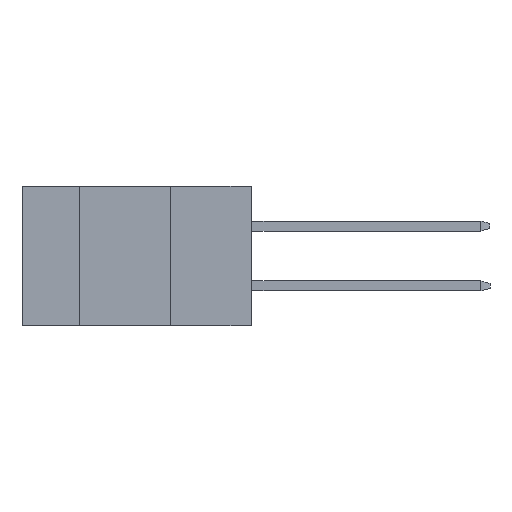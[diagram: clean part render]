
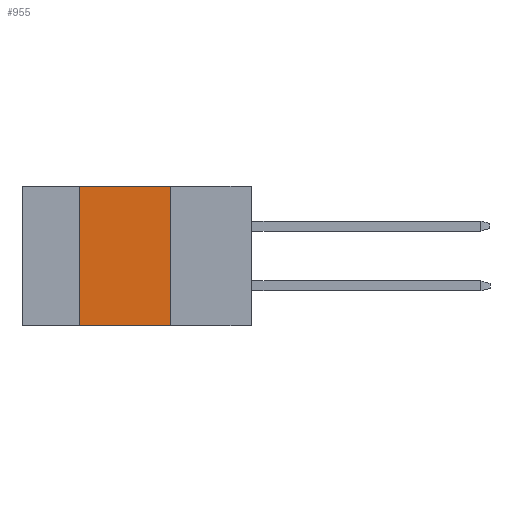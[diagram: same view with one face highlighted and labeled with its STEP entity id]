
A CAD part, left-side view. The second image highlights one B-rep face of the part: STEP entity #955.
In plain terms, the highlighted planar face has unit normal (-1, 0, 0).
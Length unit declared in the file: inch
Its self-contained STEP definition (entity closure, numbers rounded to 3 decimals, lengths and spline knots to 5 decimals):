
#553 = CARTESIAN_POINT ( 'NONE',  ( 0., 0.72, 0. ) ) ;
#832 = CARTESIAN_POINT ( 'NONE',  ( 0., 0.54, 0. ) ) ;
#886 = ORIENTED_EDGE ( 'NONE', *, *, #18858, .F. ) ;
#948 = VECTOR ( 'NONE', #7452, 39.37008 ) ;
#955 = ADVANCED_FACE ( 'NONE', ( #5339 ), #12998, .F. ) ;
#1209 = VECTOR ( 'NONE', #9947, 39.37008 ) ;
#1805 = CARTESIAN_POINT ( 'NONE',  ( 0., 0.72, -0.437 ) ) ;
#2379 = DIRECTION ( 'NONE',  ( 0., 0., -1. ) ) ;
#3817 = DIRECTION ( 'NONE',  ( 1., 0., 0. ) ) ;
#5339 = FACE_OUTER_BOUND ( 'NONE', #17587, .T. ) ;
#6115 = LINE ( 'NONE', #17029, #948 ) ;
#6169 = CARTESIAN_POINT ( 'NONE',  ( 0., 0.254, -0.437 ) ) ;
#6450 = CARTESIAN_POINT ( 'NONE',  ( 0., 0.254, 0. ) ) ;
#6986 = ORIENTED_EDGE ( 'NONE', *, *, #19279, .F. ) ;
#7402 = CARTESIAN_POINT ( 'NONE',  ( 0., 0.54, -0.437 ) ) ;
#7452 = DIRECTION ( 'NONE',  ( 0., 0., 1. ) ) ;
#7473 = DIRECTION ( 'NONE',  ( 0., 0., -1. ) ) ;
#8371 = AXIS2_PLACEMENT_3D ( 'NONE', #13296, #3817, #2379 ) ;
#8615 = EDGE_CURVE ( 'NONE', #10227, #19794, #9450, .T. ) ;
#8913 = CARTESIAN_POINT ( 'NONE',  ( 0., 0.254, -0.437 ) ) ;
#9450 = LINE ( 'NONE', #1805, #16130 ) ;
#9947 = DIRECTION ( 'NONE',  ( 0., -1., 0. ) ) ;
#10227 = VERTEX_POINT ( 'NONE', #7402 ) ;
#10707 = ORIENTED_EDGE ( 'NONE', *, *, #17778, .F. ) ;
#11055 = VERTEX_POINT ( 'NONE', #6450 ) ;
#12347 = VECTOR ( 'NONE', #7473, 39.37008 ) ;
#12717 = VERTEX_POINT ( 'NONE', #832 ) ;
#12998 = PLANE ( 'NONE',  #8371 ) ;
#13296 = CARTESIAN_POINT ( 'NONE',  ( 0., 0.72, 0. ) ) ;
#14045 = DIRECTION ( 'NONE',  ( 0., -1., 0. ) ) ;
#14528 = LINE ( 'NONE', #553, #1209 ) ;
#15838 = ORIENTED_EDGE ( 'NONE', *, *, #8615, .T. ) ;
#16130 = VECTOR ( 'NONE', #14045, 39.37008 ) ;
#16659 = LINE ( 'NONE', #8913, #12347 ) ;
#17029 = CARTESIAN_POINT ( 'NONE',  ( 0., 0.54, -0.437 ) ) ;
#17587 = EDGE_LOOP ( 'NONE', ( #886, #10707, #6986, #15838 ) ) ;
#17778 = EDGE_CURVE ( 'NONE', #12717, #11055, #14528, .T. ) ;
#18858 = EDGE_CURVE ( 'NONE', #11055, #19794, #16659, .T. ) ;
#19279 = EDGE_CURVE ( 'NONE', #10227, #12717, #6115, .T. ) ;
#19794 = VERTEX_POINT ( 'NONE', #6169 ) ;
